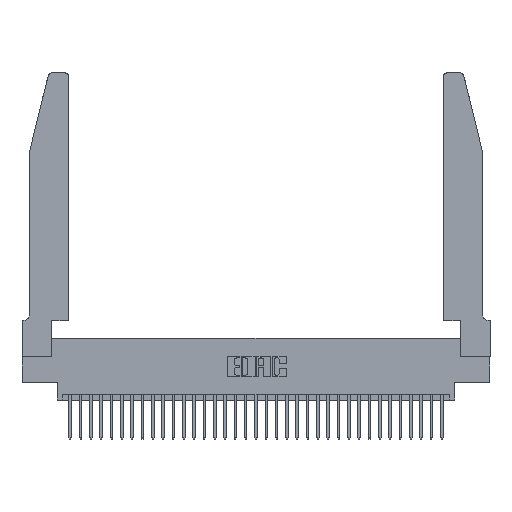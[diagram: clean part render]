
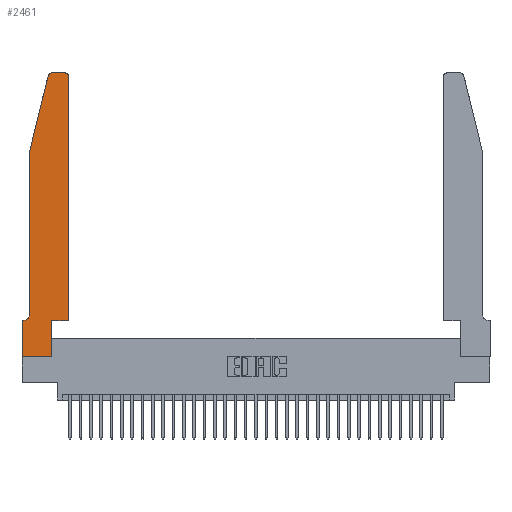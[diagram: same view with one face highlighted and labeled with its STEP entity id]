
A CAD part, top view. The second image highlights one B-rep face of the part: STEP entity #2461.
In plain terms, the highlighted planar face has unit normal (0, 0, 1).
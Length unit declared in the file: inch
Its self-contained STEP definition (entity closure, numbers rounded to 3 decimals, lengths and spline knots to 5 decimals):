
#38 = VERTEX_POINT ( 'NONE', #1027 ) ;
#167 = ORIENTED_EDGE ( 'NONE', *, *, #18233, .T. ) ;
#615 = VERTEX_POINT ( 'NONE', #24642 ) ;
#842 = AXIS2_PLACEMENT_3D ( 'NONE', #1111, #30504, #9314 ) ;
#1027 = CARTESIAN_POINT ( 'NONE',  ( 0.4505, 0.35, 0.37 ) ) ;
#1111 = CARTESIAN_POINT ( 'NONE',  ( 0.0055, 0.42, 0.37 ) ) ;
#1507 = LINE ( 'NONE', #20030, #19465 ) ;
#1900 = CARTESIAN_POINT ( 'NONE',  ( 0.2605, 2.75, 0.37 ) ) ;
#1934 = ORIENTED_EDGE ( 'NONE', *, *, #14379, .T. ) ;
#2394 = VERTEX_POINT ( 'NONE', #32054 ) ;
#2461 = ADVANCED_FACE ( 'NONE', ( #5122 ), #4538, .T. ) ;
#2834 = EDGE_CURVE ( 'NONE', #23979, #38, #23507, .T. ) ;
#3465 = VERTEX_POINT ( 'NONE', #32463 ) ;
#3554 = CARTESIAN_POINT ( 'NONE',  ( 0.2865, 0., 0.37 ) ) ;
#3798 = ORIENTED_EDGE ( 'NONE', *, *, #4235, .T. ) ;
#4235 = EDGE_CURVE ( 'NONE', #6573, #22420, #19000, .T. ) ;
#4538 = PLANE ( 'NONE',  #5266 ) ;
#4884 = DIRECTION ( 'NONE',  ( 1., 0., 0. ) ) ;
#5008 = EDGE_CURVE ( 'NONE', #30972, #32216, #7739, .T. ) ;
#5122 = FACE_OUTER_BOUND ( 'NONE', #7888, .T. ) ;
#5266 = AXIS2_PLACEMENT_3D ( 'NONE', #31568, #33754, #4884 ) ;
#6573 = VERTEX_POINT ( 'NONE', #14208 ) ;
#6611 = CARTESIAN_POINT ( 'NONE',  ( 0.4505, 0.35, 0.37 ) ) ;
#6861 = EDGE_CURVE ( 'NONE', #38, #26284, #22186, .T. ) ;
#7073 = DIRECTION ( 'NONE',  ( -0.239, -0.971, 0. ) ) ;
#7648 = VECTOR ( 'NONE', #24048, 39.37008 ) ;
#7739 = CIRCLE ( 'NONE', #23436, 0.03 ) ;
#7888 = EDGE_LOOP ( 'NONE', ( #9588, #8321, #17393, #167, #28112, #3798, #13804, #27038, #1934, #29685, #30042, #9110 ) ) ;
#8046 = VECTOR ( 'NONE', #17920, 39.37008 ) ;
#8058 = CARTESIAN_POINT ( 'NONE',  ( 0.0755, 0.35, 0.37 ) ) ;
#8321 = ORIENTED_EDGE ( 'NONE', *, *, #5008, .T. ) ;
#8778 = LINE ( 'NONE', #1900, #33501 ) ;
#8833 = DIRECTION ( 'NONE',  ( 1., 0., 0. ) ) ;
#8947 = VECTOR ( 'NONE', #13358, 39.37008 ) ;
#8948 = VECTOR ( 'NONE', #22613, 39.37008 ) ;
#9110 = ORIENTED_EDGE ( 'NONE', *, *, #32750, .T. ) ;
#9135 = EDGE_CURVE ( 'NONE', #615, #6573, #29607, .T. ) ;
#9314 = DIRECTION ( 'NONE',  ( -1., 0., 0. ) ) ;
#9588 = ORIENTED_EDGE ( 'NONE', *, *, #19268, .T. ) ;
#9620 = DIRECTION ( 'NONE',  ( -1., 0., 0. ) ) ;
#10920 = DIRECTION ( 'NONE',  ( 0., 1., 0. ) ) ;
#12094 = DIRECTION ( 'NONE',  ( 1., 0., 0. ) ) ;
#13083 = LINE ( 'NONE', #17690, #7648 ) ;
#13358 = DIRECTION ( 'NONE',  ( -1., 0., 0. ) ) ;
#13804 = ORIENTED_EDGE ( 'NONE', *, *, #17701, .T. ) ;
#13880 = VECTOR ( 'NONE', #12094, 39.37008 ) ;
#14208 = CARTESIAN_POINT ( 'NONE',  ( 0.0055, 0.35, 0.37 ) ) ;
#14379 = EDGE_CURVE ( 'NONE', #14632, #23979, #28259, .T. ) ;
#14493 = CARTESIAN_POINT ( 'NONE',  ( 0.0755, 2., 0.37 ) ) ;
#14632 = VERTEX_POINT ( 'NONE', #3554 ) ;
#15229 = CARTESIAN_POINT ( 'NONE',  ( 0.2865, 0.35, 0.37 ) ) ;
#15599 = DIRECTION ( 'NONE',  ( 0., 0., 1. ) ) ;
#17189 = DIRECTION ( 'NONE',  ( 0., -1., 0. ) ) ;
#17301 = CARTESIAN_POINT ( 'NONE',  ( 0.2865, 0.35, 0.37 ) ) ;
#17393 = ORIENTED_EDGE ( 'NONE', *, *, #22658, .T. ) ;
#17690 = CARTESIAN_POINT ( 'NONE',  ( 0., 0., 0.37 ) ) ;
#17701 = EDGE_CURVE ( 'NONE', #22420, #30271, #23172, .T. ) ;
#17920 = DIRECTION ( 'NONE',  ( 0., -1., 0. ) ) ;
#18233 = EDGE_CURVE ( 'NONE', #2394, #615, #25617, .T. ) ;
#18564 = EDGE_CURVE ( 'NONE', #30271, #14632, #13083, .T. ) ;
#19000 = LINE ( 'NONE', #8058, #8947 ) ;
#19268 = EDGE_CURVE ( 'NONE', #3465, #30972, #8778, .T. ) ;
#19365 = DIRECTION ( 'NONE',  ( 0., 0., 1. ) ) ;
#19465 = VECTOR ( 'NONE', #7073, 39.37008 ) ;
#20030 = CARTESIAN_POINT ( 'NONE',  ( 0.0755, 2., 0.37 ) ) ;
#20203 = CARTESIAN_POINT ( 'NONE',  ( 0., 0., 0.37 ) ) ;
#20323 = CARTESIAN_POINT ( 'NONE',  ( 0., 0.35, 0.37 ) ) ;
#21396 = VECTOR ( 'NONE', #10920, 39.37008 ) ;
#21819 = CARTESIAN_POINT ( 'NONE',  ( 0.284, 2.72, 0.37 ) ) ;
#22186 = LINE ( 'NONE', #26952, #21396 ) ;
#22407 = CARTESIAN_POINT ( 'NONE',  ( 0., 0., 0.37 ) ) ;
#22420 = VERTEX_POINT ( 'NONE', #20323 ) ;
#22613 = DIRECTION ( 'NONE',  ( 0., 1., 0. ) ) ;
#22658 = EDGE_CURVE ( 'NONE', #32216, #2394, #1507, .T. ) ;
#22723 = VECTOR ( 'NONE', #17189, 39.37008 ) ;
#23172 = LINE ( 'NONE', #20203, #22723 ) ;
#23272 = CARTESIAN_POINT ( 'NONE',  ( 0.4205, 2.72, 0.37 ) ) ;
#23436 = AXIS2_PLACEMENT_3D ( 'NONE', #21819, #19365, #8833 ) ;
#23507 = LINE ( 'NONE', #6611, #13880 ) ;
#23590 = CARTESIAN_POINT ( 'NONE',  ( 0.4505, 2.72, 0.37 ) ) ;
#23979 = VERTEX_POINT ( 'NONE', #15229 ) ;
#24048 = DIRECTION ( 'NONE',  ( 1., 0., 0. ) ) ;
#24642 = CARTESIAN_POINT ( 'NONE',  ( 0.0755, 0.42, 0.37 ) ) ;
#25283 = CARTESIAN_POINT ( 'NONE',  ( 0.284, 2.75, 0.37 ) ) ;
#25617 = LINE ( 'NONE', #14493, #8046 ) ;
#26284 = VERTEX_POINT ( 'NONE', #23590 ) ;
#26952 = CARTESIAN_POINT ( 'NONE',  ( 0.4505, 0.35, 0.37 ) ) ;
#27038 = ORIENTED_EDGE ( 'NONE', *, *, #18564, .T. ) ;
#28112 = ORIENTED_EDGE ( 'NONE', *, *, #9135, .T. ) ;
#28259 = LINE ( 'NONE', #17301, #8948 ) ;
#29607 = CIRCLE ( 'NONE', #842, 0.07 ) ;
#29685 = ORIENTED_EDGE ( 'NONE', *, *, #2834, .T. ) ;
#30042 = ORIENTED_EDGE ( 'NONE', *, *, #6861, .T. ) ;
#30271 = VERTEX_POINT ( 'NONE', #22407 ) ;
#30504 = DIRECTION ( 'NONE',  ( 0., 0., -1. ) ) ;
#30972 = VERTEX_POINT ( 'NONE', #25283 ) ;
#31568 = CARTESIAN_POINT ( 'NONE',  ( 0., 0.35, 0.37 ) ) ;
#32054 = CARTESIAN_POINT ( 'NONE',  ( 0.0755, 2., 0.37 ) ) ;
#32216 = VERTEX_POINT ( 'NONE', #34397 ) ;
#32462 = CIRCLE ( 'NONE', #32978, 0.03 ) ;
#32463 = CARTESIAN_POINT ( 'NONE',  ( 0.4205, 2.75, 0.37 ) ) ;
#32750 = EDGE_CURVE ( 'NONE', #26284, #3465, #32462, .T. ) ;
#32978 = AXIS2_PLACEMENT_3D ( 'NONE', #23272, #15599, #33782 ) ;
#33501 = VECTOR ( 'NONE', #9620, 39.37008 ) ;
#33754 = DIRECTION ( 'NONE',  ( 0., 0., 1. ) ) ;
#33782 = DIRECTION ( 'NONE',  ( 1., 0., 0. ) ) ;
#34397 = CARTESIAN_POINT ( 'NONE',  ( 0.25487, 2.72718, 0.37 ) ) ;
